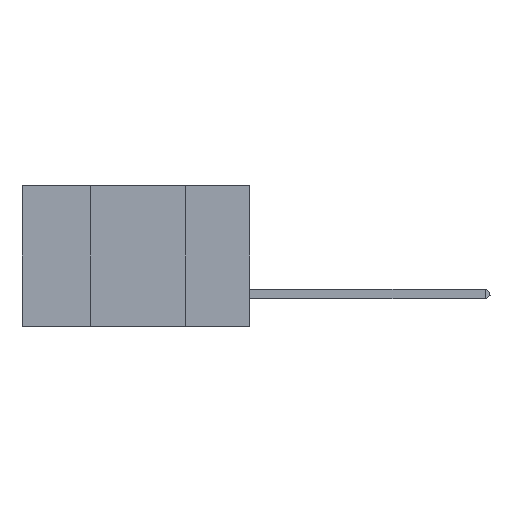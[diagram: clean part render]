
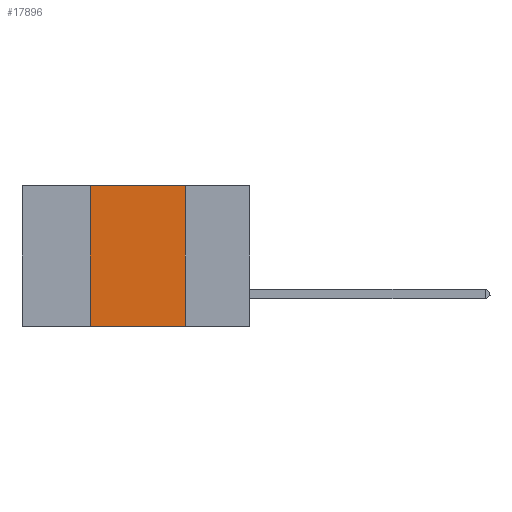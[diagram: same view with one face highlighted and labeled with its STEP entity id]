
A CAD part, left-side view. The second image highlights one B-rep face of the part: STEP entity #17896.
In plain terms, the highlighted planar face has unit normal (-1, 0, 0).
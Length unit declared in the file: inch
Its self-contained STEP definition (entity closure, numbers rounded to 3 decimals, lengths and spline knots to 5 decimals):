
#229 = DIRECTION ( 'NONE',  ( 0., 0., -1. ) ) ;
#2646 = CARTESIAN_POINT ( 'NONE',  ( 0., 0.42, 0. ) ) ;
#4687 = LINE ( 'NONE', #2646, #42861 ) ;
#5639 = DIRECTION ( 'NONE',  ( 0., -1., 0. ) ) ;
#7877 = EDGE_CURVE ( 'NONE', #8622, #22471, #4687, .T. ) ;
#8622 = VERTEX_POINT ( 'NONE', #27206 ) ;
#8892 = EDGE_LOOP ( 'NONE', ( #30334, #23394, #28429, #29167 ) ) ;
#10172 = PLANE ( 'NONE',  #24749 ) ;
#11790 = VECTOR ( 'NONE', #29840, 39.37008 ) ;
#12568 = LINE ( 'NONE', #36229, #33628 ) ;
#13143 = CARTESIAN_POINT ( 'NONE',  ( 0., 0.42, 0. ) ) ;
#15818 = EDGE_CURVE ( 'NONE', #24740, #26947, #43634, .T. ) ;
#17896 = ADVANCED_FACE ( 'NONE', ( #31008 ), #10172, .F. ) ;
#19333 = CARTESIAN_POINT ( 'NONE',  ( 0., 0.17, 0. ) ) ;
#19339 = DIRECTION ( 'NONE',  ( 0., 0., 1. ) ) ;
#20850 = VECTOR ( 'NONE', #5639, 39.37008 ) ;
#22471 = VERTEX_POINT ( 'NONE', #13143 ) ;
#23394 = ORIENTED_EDGE ( 'NONE', *, *, #25054, .F. ) ;
#23798 = CARTESIAN_POINT ( 'NONE',  ( 0., 0.6, -0.37 ) ) ;
#24740 = VERTEX_POINT ( 'NONE', #31578 ) ;
#24749 = AXIS2_PLACEMENT_3D ( 'NONE', #27425, #27427, #229 ) ;
#25054 = EDGE_CURVE ( 'NONE', #22471, #24740, #12568, .T. ) ;
#25393 = LINE ( 'NONE', #23798, #20850 ) ;
#26947 = VERTEX_POINT ( 'NONE', #39244 ) ;
#27206 = CARTESIAN_POINT ( 'NONE',  ( 0., 0.42, -0.37 ) ) ;
#27425 = CARTESIAN_POINT ( 'NONE',  ( 0., 0.6, 0. ) ) ;
#27427 = DIRECTION ( 'NONE',  ( 1., 0., 0. ) ) ;
#28429 = ORIENTED_EDGE ( 'NONE', *, *, #7877, .F. ) ;
#29167 = ORIENTED_EDGE ( 'NONE', *, *, #32358, .T. ) ;
#29840 = DIRECTION ( 'NONE',  ( 0., 0., -1. ) ) ;
#30334 = ORIENTED_EDGE ( 'NONE', *, *, #15818, .F. ) ;
#31008 = FACE_OUTER_BOUND ( 'NONE', #8892, .T. ) ;
#31578 = CARTESIAN_POINT ( 'NONE',  ( 0., 0.17, 0. ) ) ;
#32358 = EDGE_CURVE ( 'NONE', #8622, #26947, #25393, .T. ) ;
#33628 = VECTOR ( 'NONE', #43744, 39.37008 ) ;
#36229 = CARTESIAN_POINT ( 'NONE',  ( 0., 0.6, 0. ) ) ;
#39244 = CARTESIAN_POINT ( 'NONE',  ( 0., 0.17, -0.37 ) ) ;
#42861 = VECTOR ( 'NONE', #19339, 39.37008 ) ;
#43634 = LINE ( 'NONE', #19333, #11790 ) ;
#43744 = DIRECTION ( 'NONE',  ( 0., -1., 0. ) ) ;
